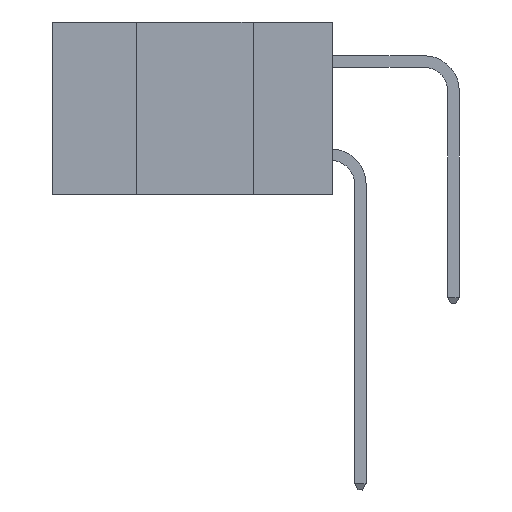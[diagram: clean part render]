
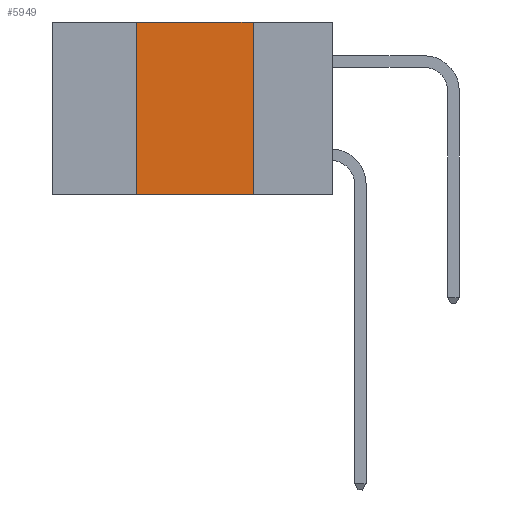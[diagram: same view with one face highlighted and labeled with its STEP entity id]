
A CAD part, left-side view. The second image highlights one B-rep face of the part: STEP entity #5949.
In plain terms, the highlighted planar face has unit normal (-1, 0, 0).
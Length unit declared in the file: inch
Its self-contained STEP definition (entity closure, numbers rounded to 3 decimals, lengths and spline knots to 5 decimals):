
#37 = DIRECTION ( 'NONE',  ( 0., -1., 0. ) ) ;
#1285 = VERTEX_POINT ( 'NONE', #14488 ) ;
#1837 = VECTOR ( 'NONE', #17759, 39.37008 ) ;
#2119 = CARTESIAN_POINT ( 'NONE',  ( 0., 0.17, 0. ) ) ;
#2474 = DIRECTION ( 'NONE',  ( 0., 0., -1. ) ) ;
#4674 = DIRECTION ( 'NONE',  ( 0., 0., -1. ) ) ;
#5949 = ADVANCED_FACE ( 'NONE', ( #16286 ), #6161, .F. ) ;
#6161 = PLANE ( 'NONE',  #20248 ) ;
#7159 = VECTOR ( 'NONE', #19828, 39.37008 ) ;
#7831 = LINE ( 'NONE', #15947, #7159 ) ;
#7903 = CARTESIAN_POINT ( 'NONE',  ( 0., 0.42, -0.37 ) ) ;
#9512 = ORIENTED_EDGE ( 'NONE', *, *, #16821, .F. ) ;
#10521 = CARTESIAN_POINT ( 'NONE',  ( 0., 0.17, -0.37 ) ) ;
#10950 = DIRECTION ( 'NONE',  ( 1., 0., 0. ) ) ;
#11976 = LINE ( 'NONE', #18223, #17036 ) ;
#12312 = EDGE_LOOP ( 'NONE', ( #12339, #25555, #9512, #22553 ) ) ;
#12339 = ORIENTED_EDGE ( 'NONE', *, *, #19028, .F. ) ;
#12362 = EDGE_CURVE ( 'NONE', #13199, #18861, #11976, .T. ) ;
#13199 = VERTEX_POINT ( 'NONE', #13244 ) ;
#13244 = CARTESIAN_POINT ( 'NONE',  ( 0., 0.42, -0.37 ) ) ;
#13486 = LINE ( 'NONE', #7903, #1837 ) ;
#14488 = CARTESIAN_POINT ( 'NONE',  ( 0., 0.42, 0. ) ) ;
#15947 = CARTESIAN_POINT ( 'NONE',  ( 0., 0.6, 0. ) ) ;
#16286 = FACE_OUTER_BOUND ( 'NONE', #12312, .T. ) ;
#16821 = EDGE_CURVE ( 'NONE', #13199, #1285, #13486, .T. ) ;
#17036 = VECTOR ( 'NONE', #37, 39.37008 ) ;
#17759 = DIRECTION ( 'NONE',  ( 0., 0., 1. ) ) ;
#18223 = CARTESIAN_POINT ( 'NONE',  ( 0., 0.6, -0.37 ) ) ;
#18487 = VECTOR ( 'NONE', #2474, 39.37008 ) ;
#18861 = VERTEX_POINT ( 'NONE', #10521 ) ;
#19028 = EDGE_CURVE ( 'NONE', #20863, #18861, #23051, .T. ) ;
#19828 = DIRECTION ( 'NONE',  ( 0., -1., 0. ) ) ;
#20248 = AXIS2_PLACEMENT_3D ( 'NONE', #21341, #10950, #4674 ) ;
#20863 = VERTEX_POINT ( 'NONE', #2119 ) ;
#21030 = CARTESIAN_POINT ( 'NONE',  ( 0., 0.17, -0.37 ) ) ;
#21341 = CARTESIAN_POINT ( 'NONE',  ( 0., 0.6, 0. ) ) ;
#22553 = ORIENTED_EDGE ( 'NONE', *, *, #12362, .T. ) ;
#23051 = LINE ( 'NONE', #21030, #18487 ) ;
#24801 = EDGE_CURVE ( 'NONE', #1285, #20863, #7831, .T. ) ;
#25555 = ORIENTED_EDGE ( 'NONE', *, *, #24801, .F. ) ;
